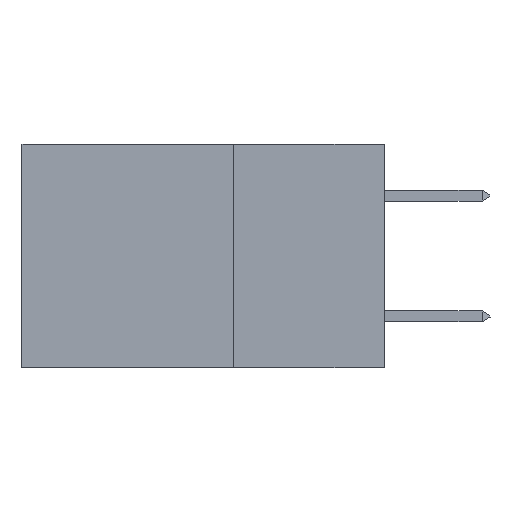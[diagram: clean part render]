
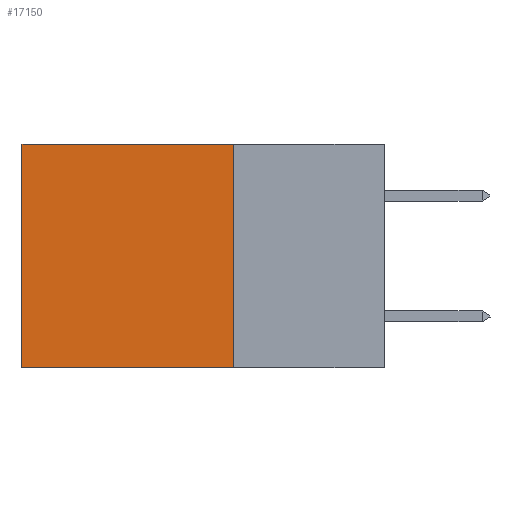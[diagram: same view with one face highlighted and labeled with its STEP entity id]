
A CAD part, left-side view. The second image highlights one B-rep face of the part: STEP entity #17150.
In plain terms, the highlighted planar face has unit normal (-1, 0, 0).
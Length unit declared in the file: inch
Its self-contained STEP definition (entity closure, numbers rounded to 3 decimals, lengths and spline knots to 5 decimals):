
#919 = DIRECTION ( 'NONE',  ( 1., 0., 0. ) ) ;
#969 = EDGE_CURVE ( 'NONE', #4673, #17287, #22988, .T. ) ;
#1135 = CARTESIAN_POINT ( 'NONE',  ( 0.2875, 0.6, -0.37 ) ) ;
#2137 = CARTESIAN_POINT ( 'NONE',  ( 0.2875, 0.6, 0. ) ) ;
#2371 = AXIS2_PLACEMENT_3D ( 'NONE', #15543, #919, #4458 ) ;
#3328 = VECTOR ( 'NONE', #6757, 39.37008 ) ;
#3618 = CARTESIAN_POINT ( 'NONE',  ( 0.2875, 0.25, 0. ) ) ;
#4458 = DIRECTION ( 'NONE',  ( 0., 0., -1. ) ) ;
#4673 = VERTEX_POINT ( 'NONE', #2137 ) ;
#4853 = EDGE_CURVE ( 'NONE', #13013, #4673, #5894, .T. ) ;
#4923 = EDGE_CURVE ( 'NONE', #13013, #16491, #12257, .T. ) ;
#5186 = CARTESIAN_POINT ( 'NONE',  ( 0.2875, 0.25, 0. ) ) ;
#5894 = LINE ( 'NONE', #3618, #9642 ) ;
#6295 = VECTOR ( 'NONE', #22150, 39.37008 ) ;
#6757 = DIRECTION ( 'NONE',  ( 0., 1., 0. ) ) ;
#6826 = LINE ( 'NONE', #17507, #3328 ) ;
#7167 = CARTESIAN_POINT ( 'NONE',  ( 0.2875, 0.25, -0.37 ) ) ;
#9580 = ORIENTED_EDGE ( 'NONE', *, *, #4923, .F. ) ;
#9642 = VECTOR ( 'NONE', #14851, 39.37008 ) ;
#12257 = LINE ( 'NONE', #20222, #21447 ) ;
#13013 = VERTEX_POINT ( 'NONE', #5186 ) ;
#14730 = ORIENTED_EDGE ( 'NONE', *, *, #969, .T. ) ;
#14851 = DIRECTION ( 'NONE',  ( 0., 1., 0. ) ) ;
#15214 = EDGE_CURVE ( 'NONE', #16491, #17287, #6826, .T. ) ;
#15381 = ORIENTED_EDGE ( 'NONE', *, *, #15214, .F. ) ;
#15543 = CARTESIAN_POINT ( 'NONE',  ( 0.2875, 0.25, 0. ) ) ;
#15696 = PLANE ( 'NONE',  #2371 ) ;
#16491 = VERTEX_POINT ( 'NONE', #7167 ) ;
#17150 = ADVANCED_FACE ( 'NONE', ( #23565 ), #15696, .F. ) ;
#17287 = VERTEX_POINT ( 'NONE', #1135 ) ;
#17507 = CARTESIAN_POINT ( 'NONE',  ( 0.2875, 0.25, -0.37 ) ) ;
#18566 = EDGE_LOOP ( 'NONE', ( #14730, #15381, #9580, #19004 ) ) ;
#18729 = DIRECTION ( 'NONE',  ( 0., 0., -1. ) ) ;
#19004 = ORIENTED_EDGE ( 'NONE', *, *, #4853, .T. ) ;
#20222 = CARTESIAN_POINT ( 'NONE',  ( 0.2875, 0.25, 0. ) ) ;
#20301 = CARTESIAN_POINT ( 'NONE',  ( 0.2875, 0.6, 0. ) ) ;
#21447 = VECTOR ( 'NONE', #18729, 39.37008 ) ;
#22150 = DIRECTION ( 'NONE',  ( 0., 0., -1. ) ) ;
#22988 = LINE ( 'NONE', #20301, #6295 ) ;
#23565 = FACE_OUTER_BOUND ( 'NONE', #18566, .T. ) ;
